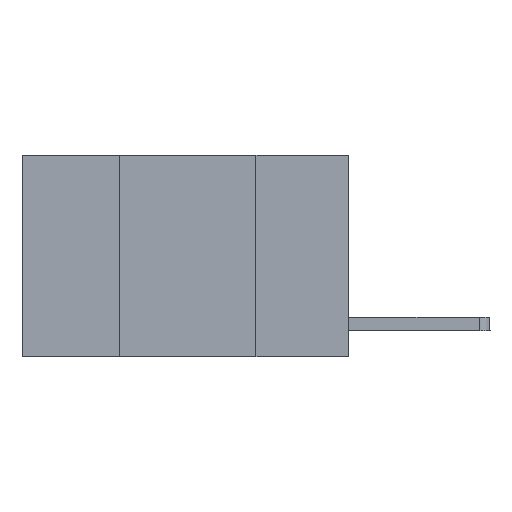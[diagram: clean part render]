
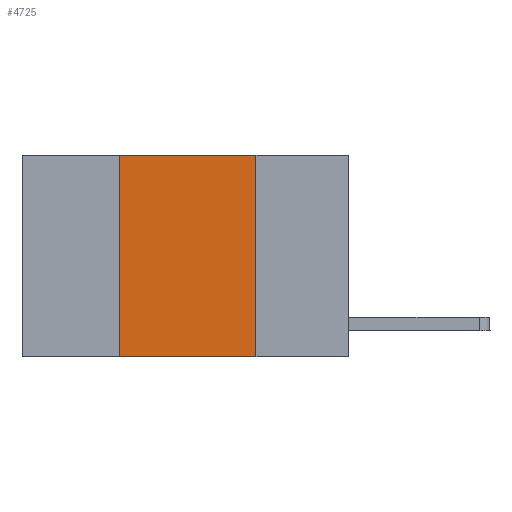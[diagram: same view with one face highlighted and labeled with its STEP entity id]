
A CAD part, left-side view. The second image highlights one B-rep face of the part: STEP entity #4725.
In plain terms, the highlighted planar face has unit normal (-1, 0, 0).
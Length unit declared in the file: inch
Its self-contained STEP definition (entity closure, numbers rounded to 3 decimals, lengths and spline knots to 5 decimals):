
#163 = EDGE_LOOP ( 'NONE', ( #8051, #2756, #389, #6759 ) ) ;
#380 = DIRECTION ( 'NONE',  ( 0., -1., 0. ) ) ;
#389 = ORIENTED_EDGE ( 'NONE', *, *, #9710, .F. ) ;
#770 = LINE ( 'NONE', #6988, #5122 ) ;
#838 = DIRECTION ( 'NONE',  ( 1., 0., 0. ) ) ;
#954 = CARTESIAN_POINT ( 'NONE',  ( 0., 0.42, -0.37 ) ) ;
#1483 = DIRECTION ( 'NONE',  ( 0., -1., 0. ) ) ;
#1516 = FACE_OUTER_BOUND ( 'NONE', #163, .T. ) ;
#2268 = CARTESIAN_POINT ( 'NONE',  ( 0., 0.6, 0. ) ) ;
#2756 = ORIENTED_EDGE ( 'NONE', *, *, #4146, .F. ) ;
#2939 = VECTOR ( 'NONE', #5225, 39.37008 ) ;
#3160 = CARTESIAN_POINT ( 'NONE',  ( 0., 0.6, -0.37 ) ) ;
#3291 = VERTEX_POINT ( 'NONE', #954 ) ;
#3374 = EDGE_CURVE ( 'NONE', #8433, #3957, #7545, .T. ) ;
#3443 = VECTOR ( 'NONE', #1483, 39.37008 ) ;
#3957 = VERTEX_POINT ( 'NONE', #8452 ) ;
#3994 = DIRECTION ( 'NONE',  ( 0., 0., 1. ) ) ;
#4146 = EDGE_CURVE ( 'NONE', #6003, #8433, #4479, .T. ) ;
#4479 = LINE ( 'NONE', #5335, #3443 ) ;
#4673 = CARTESIAN_POINT ( 'NONE',  ( 0., 0.42, 0. ) ) ;
#4725 = ADVANCED_FACE ( 'NONE', ( #1516 ), #7753, .F. ) ;
#5122 = VECTOR ( 'NONE', #3994, 39.37008 ) ;
#5225 = DIRECTION ( 'NONE',  ( 0., 0., -1. ) ) ;
#5335 = CARTESIAN_POINT ( 'NONE',  ( 0., 0.6, 0. ) ) ;
#6003 = VERTEX_POINT ( 'NONE', #4673 ) ;
#6036 = EDGE_CURVE ( 'NONE', #3291, #3957, #8572, .T. ) ;
#6160 = CARTESIAN_POINT ( 'NONE',  ( 0., 0.17, 0. ) ) ;
#6660 = AXIS2_PLACEMENT_3D ( 'NONE', #2268, #838, #7798 ) ;
#6759 = ORIENTED_EDGE ( 'NONE', *, *, #6036, .T. ) ;
#6988 = CARTESIAN_POINT ( 'NONE',  ( 0., 0.42, 0. ) ) ;
#7545 = LINE ( 'NONE', #8159, #2939 ) ;
#7753 = PLANE ( 'NONE',  #6660 ) ;
#7798 = DIRECTION ( 'NONE',  ( 0., 0., -1. ) ) ;
#8051 = ORIENTED_EDGE ( 'NONE', *, *, #3374, .F. ) ;
#8159 = CARTESIAN_POINT ( 'NONE',  ( 0., 0.17, 0. ) ) ;
#8433 = VERTEX_POINT ( 'NONE', #6160 ) ;
#8452 = CARTESIAN_POINT ( 'NONE',  ( 0., 0.17, -0.37 ) ) ;
#8572 = LINE ( 'NONE', #3160, #8836 ) ;
#8836 = VECTOR ( 'NONE', #380, 39.37008 ) ;
#9710 = EDGE_CURVE ( 'NONE', #3291, #6003, #770, .T. ) ;
